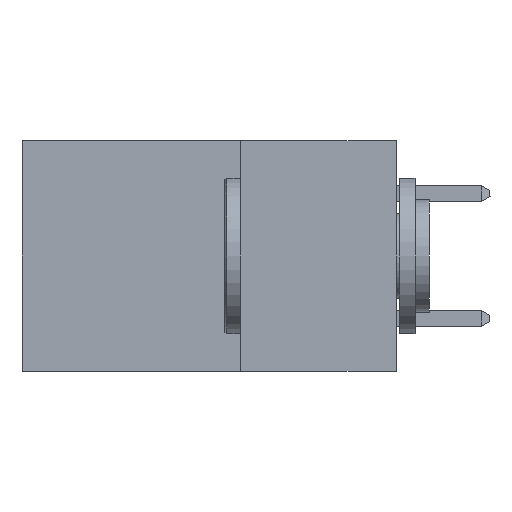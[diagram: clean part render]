
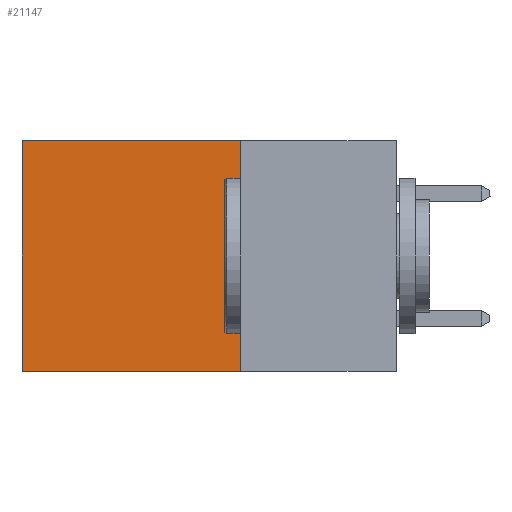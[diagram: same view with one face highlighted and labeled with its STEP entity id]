
A CAD part, left-side view. The second image highlights one B-rep face of the part: STEP entity #21147.
In plain terms, the highlighted planar face has unit normal (-1, 0, 0).
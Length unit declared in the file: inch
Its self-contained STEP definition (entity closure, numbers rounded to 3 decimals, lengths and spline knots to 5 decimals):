
#1194 = FACE_OUTER_BOUND ( 'NONE', #16798, .T. ) ;
#1267 = CARTESIAN_POINT ( 'NONE',  ( 0.298, 0.6, 0. ) ) ;
#1574 = LINE ( 'NONE', #1267, #18637 ) ;
#1588 = PLANE ( 'NONE',  #6941 ) ;
#1775 = CARTESIAN_POINT ( 'NONE',  ( 0.298, 0.25, 0. ) ) ;
#1929 = DIRECTION ( 'NONE',  ( 0., 1., 0. ) ) ;
#1934 = EDGE_CURVE ( 'NONE', #27383, #17908, #1574, .T. ) ;
#2559 = CARTESIAN_POINT ( 'NONE',  ( 0.298, 0.25, 0. ) ) ;
#3409 = DIRECTION ( 'NONE',  ( 0., 0., -1. ) ) ;
#3971 = CARTESIAN_POINT ( 'NONE',  ( 0.298, 0.6, -0.37 ) ) ;
#4122 = CARTESIAN_POINT ( 'NONE',  ( 0.298, 0.25, -0.37 ) ) ;
#5489 = VECTOR ( 'NONE', #9948, 39.37008 ) ;
#5599 = EDGE_CURVE ( 'NONE', #22332, #27383, #6574, .T. ) ;
#5721 = ORIENTED_EDGE ( 'NONE', *, *, #9004, .F. ) ;
#6093 = DIRECTION ( 'NONE',  ( 0., 0., -1. ) ) ;
#6574 = LINE ( 'NONE', #9662, #5489 ) ;
#6941 = AXIS2_PLACEMENT_3D ( 'NONE', #1775, #15341, #6093 ) ;
#7022 = ORIENTED_EDGE ( 'NONE', *, *, #1934, .T. ) ;
#8308 = LINE ( 'NONE', #2559, #9007 ) ;
#9004 = EDGE_CURVE ( 'NONE', #26834, #17908, #15005, .T. ) ;
#9007 = VECTOR ( 'NONE', #11588, 39.37008 ) ;
#9662 = CARTESIAN_POINT ( 'NONE',  ( 0.298, 0.25, 0. ) ) ;
#9948 = DIRECTION ( 'NONE',  ( 0., 1., 0. ) ) ;
#10141 = EDGE_CURVE ( 'NONE', #22332, #26834, #8308, .T. ) ;
#10818 = ORIENTED_EDGE ( 'NONE', *, *, #10141, .F. ) ;
#10827 = CARTESIAN_POINT ( 'NONE',  ( 0.298, 0.25, -0.37 ) ) ;
#11588 = DIRECTION ( 'NONE',  ( 0., 0., -1. ) ) ;
#11668 = ORIENTED_EDGE ( 'NONE', *, *, #5599, .T. ) ;
#13624 = VECTOR ( 'NONE', #1929, 39.37008 ) ;
#15005 = LINE ( 'NONE', #10827, #13624 ) ;
#15341 = DIRECTION ( 'NONE',  ( 1., 0., 0. ) ) ;
#16352 = CARTESIAN_POINT ( 'NONE',  ( 0.298, 0.25, 0. ) ) ;
#16798 = EDGE_LOOP ( 'NONE', ( #7022, #5721, #10818, #11668 ) ) ;
#17908 = VERTEX_POINT ( 'NONE', #3971 ) ;
#18637 = VECTOR ( 'NONE', #3409, 39.37008 ) ;
#21147 = ADVANCED_FACE ( 'NONE', ( #1194 ), #1588, .F. ) ;
#22332 = VERTEX_POINT ( 'NONE', #16352 ) ;
#23473 = CARTESIAN_POINT ( 'NONE',  ( 0.298, 0.6, 0. ) ) ;
#26834 = VERTEX_POINT ( 'NONE', #4122 ) ;
#27383 = VERTEX_POINT ( 'NONE', #23473 ) ;
